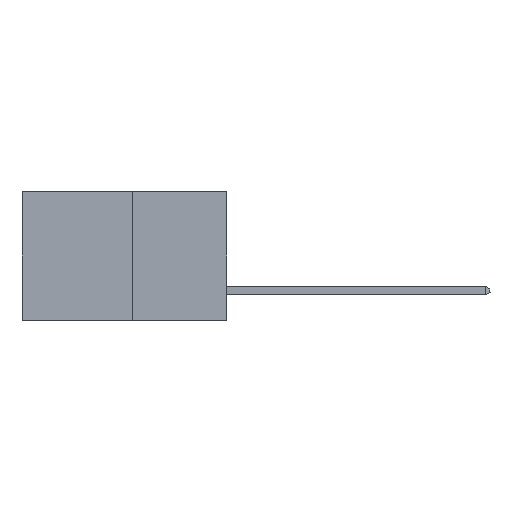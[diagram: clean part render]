
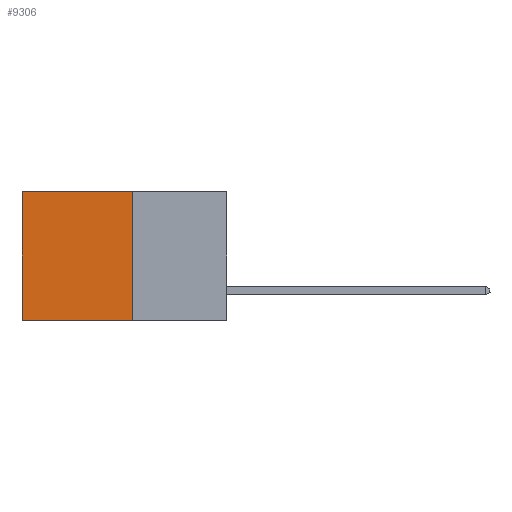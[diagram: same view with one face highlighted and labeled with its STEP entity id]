
A CAD part, left-side view. The second image highlights one B-rep face of the part: STEP entity #9306.
In plain terms, the highlighted planar face has unit normal (-1, 0, 0).
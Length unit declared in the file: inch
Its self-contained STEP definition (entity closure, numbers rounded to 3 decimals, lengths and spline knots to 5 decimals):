
#339 = CARTESIAN_POINT ( 'NONE',  ( 0.277, 0.59, 0. ) ) ;
#624 = VECTOR ( 'NONE', #893, 39.37008 ) ;
#893 = DIRECTION ( 'NONE',  ( 0., 1., 0. ) ) ;
#1178 = DIRECTION ( 'NONE',  ( 0., 0., -1. ) ) ;
#1247 = EDGE_LOOP ( 'NONE', ( #6305, #6290, #1369, #2526 ) ) ;
#1369 = ORIENTED_EDGE ( 'NONE', *, *, #5821, .F. ) ;
#1484 = VECTOR ( 'NONE', #2348, 39.37008 ) ;
#1942 = VERTEX_POINT ( 'NONE', #10236 ) ;
#2145 = EDGE_CURVE ( 'NONE', #9331, #1942, #9338, .T. ) ;
#2348 = DIRECTION ( 'NONE',  ( 0., 0., -1. ) ) ;
#2376 = CARTESIAN_POINT ( 'NONE',  ( 0.277, 0.27, -0.37 ) ) ;
#2390 = AXIS2_PLACEMENT_3D ( 'NONE', #4596, #6281, #1178 ) ;
#2526 = ORIENTED_EDGE ( 'NONE', *, *, #8119, .T. ) ;
#2885 = PLANE ( 'NONE',  #2390 ) ;
#2918 = CARTESIAN_POINT ( 'NONE',  ( 0.277, 0.27, -0.37 ) ) ;
#2947 = VECTOR ( 'NONE', #9127, 39.37008 ) ;
#3414 = LINE ( 'NONE', #9383, #5146 ) ;
#3643 = FACE_OUTER_BOUND ( 'NONE', #1247, .T. ) ;
#4596 = CARTESIAN_POINT ( 'NONE',  ( 0.277, 0.27, -0.37 ) ) ;
#4997 = CARTESIAN_POINT ( 'NONE',  ( 0.277, 0.27, 0. ) ) ;
#5146 = VECTOR ( 'NONE', #5256, 39.37008 ) ;
#5256 = DIRECTION ( 'NONE',  ( 0., 1., 0. ) ) ;
#5821 = EDGE_CURVE ( 'NONE', #8513, #9331, #7447, .T. ) ;
#6281 = DIRECTION ( 'NONE',  ( 1., 0., 0. ) ) ;
#6290 = ORIENTED_EDGE ( 'NONE', *, *, #2145, .F. ) ;
#6305 = ORIENTED_EDGE ( 'NONE', *, *, #9533, .T. ) ;
#7447 = LINE ( 'NONE', #2376, #2947 ) ;
#8078 = CARTESIAN_POINT ( 'NONE',  ( 0.277, 0.27, -0.37 ) ) ;
#8119 = EDGE_CURVE ( 'NONE', #8513, #9339, #3414, .T. ) ;
#8227 = LINE ( 'NONE', #8245, #1484 ) ;
#8245 = CARTESIAN_POINT ( 'NONE',  ( 0.277, 0.59, -0.37 ) ) ;
#8513 = VERTEX_POINT ( 'NONE', #4997 ) ;
#9127 = DIRECTION ( 'NONE',  ( 0., 0., -1. ) ) ;
#9306 = ADVANCED_FACE ( 'NONE', ( #3643 ), #2885, .F. ) ;
#9331 = VERTEX_POINT ( 'NONE', #2918 ) ;
#9338 = LINE ( 'NONE', #8078, #624 ) ;
#9339 = VERTEX_POINT ( 'NONE', #339 ) ;
#9383 = CARTESIAN_POINT ( 'NONE',  ( 0.277, 0.27, 0. ) ) ;
#9533 = EDGE_CURVE ( 'NONE', #9339, #1942, #8227, .T. ) ;
#10236 = CARTESIAN_POINT ( 'NONE',  ( 0.277, 0.59, -0.37 ) ) ;
